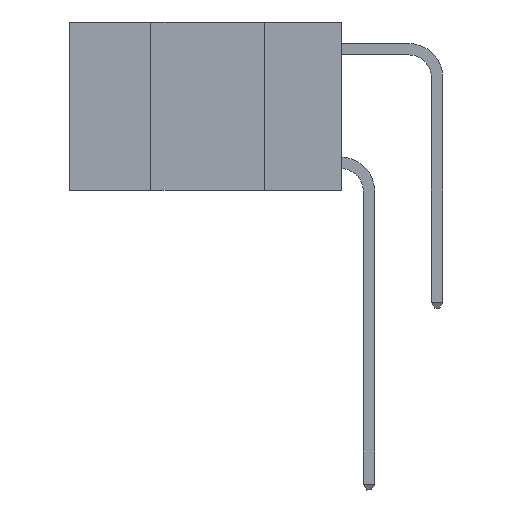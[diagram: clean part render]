
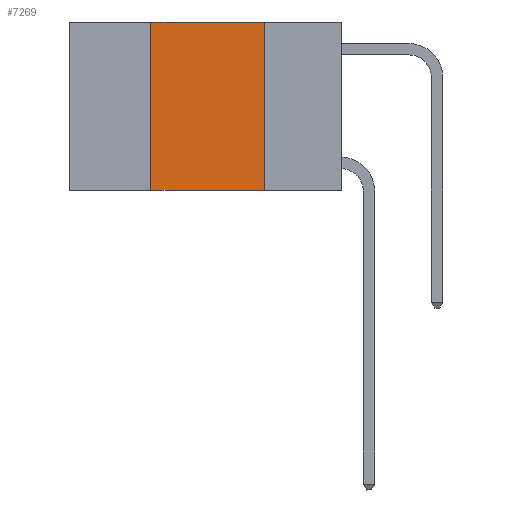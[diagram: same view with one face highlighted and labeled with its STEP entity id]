
A CAD part, left-side view. The second image highlights one B-rep face of the part: STEP entity #7269.
In plain terms, the highlighted planar face has unit normal (-1, 0, 0).
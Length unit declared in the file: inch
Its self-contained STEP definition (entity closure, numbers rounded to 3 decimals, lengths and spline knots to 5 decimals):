
#793 = EDGE_LOOP ( 'NONE', ( #20714, #3048, #3717, #15397 ) ) ;
#1238 = VERTEX_POINT ( 'NONE', #8142 ) ;
#1392 = VERTEX_POINT ( 'NONE', #20578 ) ;
#1505 = EDGE_CURVE ( 'NONE', #1392, #5784, #6028, .T. ) ;
#2559 = VECTOR ( 'NONE', #9103, 39.37008 ) ;
#3048 = ORIENTED_EDGE ( 'NONE', *, *, #10040, .F. ) ;
#3116 = CARTESIAN_POINT ( 'NONE',  ( 0., 0.17, 0. ) ) ;
#3717 = ORIENTED_EDGE ( 'NONE', *, *, #1505, .F. ) ;
#4773 = VECTOR ( 'NONE', #21227, 39.37008 ) ;
#5784 = VERTEX_POINT ( 'NONE', #15676 ) ;
#6028 = LINE ( 'NONE', #11092, #4773 ) ;
#7123 = EDGE_CURVE ( 'NONE', #13286, #1238, #21580, .T. ) ;
#7269 = ADVANCED_FACE ( 'NONE', ( #20337 ), #8455, .F. ) ;
#8142 = CARTESIAN_POINT ( 'NONE',  ( 0., 0.17, -0.37 ) ) ;
#8455 = PLANE ( 'NONE',  #21647 ) ;
#9103 = DIRECTION ( 'NONE',  ( 0., -1., 0. ) ) ;
#9893 = DIRECTION ( 'NONE',  ( 0., 0., -1. ) ) ;
#10040 = EDGE_CURVE ( 'NONE', #5784, #13286, #19659, .T. ) ;
#10207 = DIRECTION ( 'NONE',  ( 1., 0., 0. ) ) ;
#10705 = EDGE_CURVE ( 'NONE', #1392, #1238, #15049, .T. ) ;
#11092 = CARTESIAN_POINT ( 'NONE',  ( 0., 0.42, 0. ) ) ;
#11181 = CARTESIAN_POINT ( 'NONE',  ( 0., 0.6, 0. ) ) ;
#11752 = CARTESIAN_POINT ( 'NONE',  ( 0., 0.6, 0. ) ) ;
#13223 = VECTOR ( 'NONE', #19625, 39.37008 ) ;
#13286 = VERTEX_POINT ( 'NONE', #18974 ) ;
#13641 = DIRECTION ( 'NONE',  ( 0., 0., -1. ) ) ;
#15049 = LINE ( 'NONE', #18390, #13223 ) ;
#15397 = ORIENTED_EDGE ( 'NONE', *, *, #10705, .T. ) ;
#15676 = CARTESIAN_POINT ( 'NONE',  ( 0., 0.42, 0. ) ) ;
#18390 = CARTESIAN_POINT ( 'NONE',  ( 0., 0.6, -0.37 ) ) ;
#18794 = VECTOR ( 'NONE', #9893, 39.37008 ) ;
#18974 = CARTESIAN_POINT ( 'NONE',  ( 0., 0.17, 0. ) ) ;
#19625 = DIRECTION ( 'NONE',  ( 0., -1., 0. ) ) ;
#19659 = LINE ( 'NONE', #11181, #2559 ) ;
#20337 = FACE_OUTER_BOUND ( 'NONE', #793, .T. ) ;
#20578 = CARTESIAN_POINT ( 'NONE',  ( 0., 0.42, -0.37 ) ) ;
#20714 = ORIENTED_EDGE ( 'NONE', *, *, #7123, .F. ) ;
#21227 = DIRECTION ( 'NONE',  ( 0., 0., 1. ) ) ;
#21580 = LINE ( 'NONE', #3116, #18794 ) ;
#21647 = AXIS2_PLACEMENT_3D ( 'NONE', #11752, #10207, #13641 ) ;
